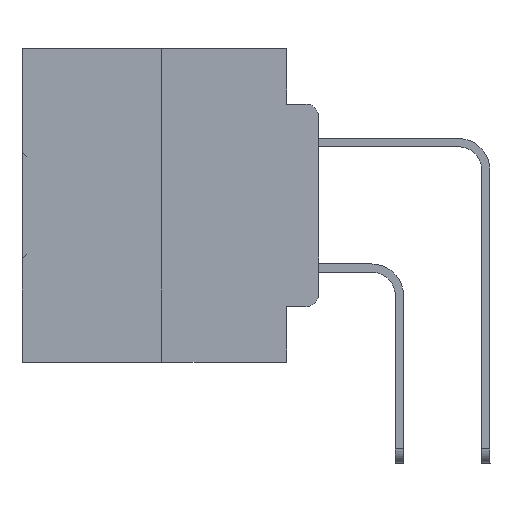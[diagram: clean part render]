
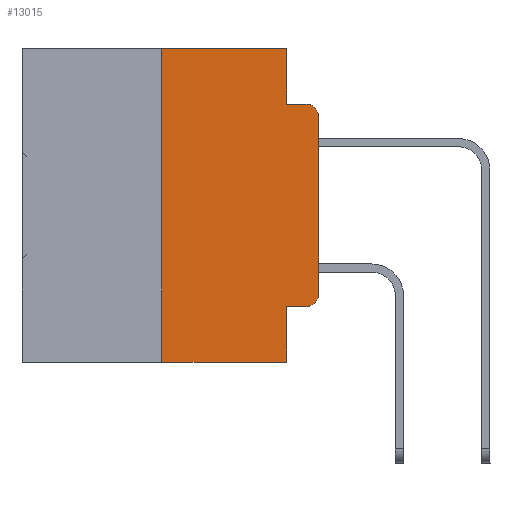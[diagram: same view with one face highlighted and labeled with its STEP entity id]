
A CAD part, left-side view. The second image highlights one B-rep face of the part: STEP entity #13015.
In plain terms, the highlighted planar face has unit normal (-1, 0, 0).
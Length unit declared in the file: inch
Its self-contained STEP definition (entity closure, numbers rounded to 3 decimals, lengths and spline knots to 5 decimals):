
#2 = LINE ( 'NONE', #14968, #14999 ) ;
#311 = DIRECTION ( 'NONE',  ( -1., 0., 0. ) ) ;
#765 = CIRCLE ( 'NONE', #27268, 0.02 ) ;
#953 = FACE_OUTER_BOUND ( 'NONE', #35140, .T. ) ;
#1009 = CARTESIAN_POINT ( 'NONE',  ( 0., 0.051, 0. ) ) ;
#1306 = CARTESIAN_POINT ( 'NONE',  ( 0., 0.051, -0.4115 ) ) ;
#2291 = LINE ( 'NONE', #12641, #8899 ) ;
#2519 = VERTEX_POINT ( 'NONE', #21751 ) ;
#3044 = VERTEX_POINT ( 'NONE', #28728 ) ;
#4275 = ORIENTED_EDGE ( 'NONE', *, *, #31903, .F. ) ;
#4675 = DIRECTION ( 'NONE',  ( 0., -1., 0. ) ) ;
#4697 = AXIS2_PLACEMENT_3D ( 'NONE', #22525, #6016, #25320 ) ;
#4734 = ORIENTED_EDGE ( 'NONE', *, *, #33663, .F. ) ;
#6016 = DIRECTION ( 'NONE',  ( 1., 0., 0. ) ) ;
#6098 = ORIENTED_EDGE ( 'NONE', *, *, #19002, .T. ) ;
#7872 = CARTESIAN_POINT ( 'NONE',  ( 0., 0.051, -0.0885 ) ) ;
#8592 = CARTESIAN_POINT ( 'NONE',  ( 0., 0.051, 0. ) ) ;
#8665 = CARTESIAN_POINT ( 'NONE',  ( 0., 0., -0.3915 ) ) ;
#8899 = VECTOR ( 'NONE', #20821, 39.37008 ) ;
#9166 = VECTOR ( 'NONE', #35363, 39.37008 ) ;
#9259 = EDGE_CURVE ( 'NONE', #13122, #3044, #13547, .T. ) ;
#10264 = CARTESIAN_POINT ( 'NONE',  ( 0., 0.473, -0.5 ) ) ;
#11190 = AXIS2_PLACEMENT_3D ( 'NONE', #17132, #311, #19896 ) ;
#11481 = CARTESIAN_POINT ( 'NONE',  ( 0., 0.02, -0.4115 ) ) ;
#11544 = PLANE ( 'NONE',  #4697 ) ;
#12348 = VECTOR ( 'NONE', #15047, 39.37008 ) ;
#12641 = CARTESIAN_POINT ( 'NONE',  ( 0., 0., 0. ) ) ;
#12862 = CIRCLE ( 'NONE', #11190, 0.02 ) ;
#13015 = ADVANCED_FACE ( 'NONE', ( #953 ), #11544, .F. ) ;
#13122 = VERTEX_POINT ( 'NONE', #1306 ) ;
#13547 = LINE ( 'NONE', #8592, #34394 ) ;
#13906 = CARTESIAN_POINT ( 'NONE',  ( 0., 0.02, -0.1085 ) ) ;
#14566 = EDGE_CURVE ( 'NONE', #28835, #17839, #17956, .T. ) ;
#14968 = CARTESIAN_POINT ( 'NONE',  ( 0., 0.473, 0. ) ) ;
#14999 = VECTOR ( 'NONE', #33939, 39.37008 ) ;
#15027 = VERTEX_POINT ( 'NONE', #11481 ) ;
#15047 = DIRECTION ( 'NONE',  ( 0., 0., -1. ) ) ;
#16044 = VERTEX_POINT ( 'NONE', #32412 ) ;
#16150 = ORIENTED_EDGE ( 'NONE', *, *, #21809, .T. ) ;
#16586 = LINE ( 'NONE', #32496, #9166 ) ;
#16682 = DIRECTION ( 'NONE',  ( 0., 0., -1. ) ) ;
#17132 = CARTESIAN_POINT ( 'NONE',  ( 0., 0.02, -0.3915 ) ) ;
#17839 = VERTEX_POINT ( 'NONE', #7872 ) ;
#17892 = ORIENTED_EDGE ( 'NONE', *, *, #33539, .T. ) ;
#17956 = LINE ( 'NONE', #1009, #12348 ) ;
#18269 = EDGE_CURVE ( 'NONE', #26277, #2519, #2291, .T. ) ;
#19002 = EDGE_CURVE ( 'NONE', #13122, #15027, #29461, .T. ) ;
#19896 = DIRECTION ( 'NONE',  ( 0., 0., -1. ) ) ;
#20504 = VERTEX_POINT ( 'NONE', #31419 ) ;
#20821 = DIRECTION ( 'NONE',  ( 0., 0., 1. ) ) ;
#21751 = CARTESIAN_POINT ( 'NONE',  ( 0., 0., -0.1085 ) ) ;
#21809 = EDGE_CURVE ( 'NONE', #16044, #3044, #35278, .T. ) ;
#21940 = EDGE_CURVE ( 'NONE', #16044, #20504, #16586, .T. ) ;
#22525 = CARTESIAN_POINT ( 'NONE',  ( 0., 0.473, 0. ) ) ;
#22625 = EDGE_CURVE ( 'NONE', #2519, #24199, #765, .T. ) ;
#23136 = VECTOR ( 'NONE', #31879, 39.37008 ) ;
#24061 = CARTESIAN_POINT ( 'NONE',  ( 0., 0.051, -0.0885 ) ) ;
#24199 = VERTEX_POINT ( 'NONE', #29444 ) ;
#24636 = ORIENTED_EDGE ( 'NONE', *, *, #22625, .T. ) ;
#25098 = DIRECTION ( 'NONE',  ( 0., 0., -1. ) ) ;
#25320 = DIRECTION ( 'NONE',  ( 0., 0., -1. ) ) ;
#25516 = ORIENTED_EDGE ( 'NONE', *, *, #9259, .F. ) ;
#26277 = VERTEX_POINT ( 'NONE', #8665 ) ;
#26313 = ORIENTED_EDGE ( 'NONE', *, *, #14566, .F. ) ;
#26567 = CARTESIAN_POINT ( 'NONE',  ( 0., 0.051, -0.4115 ) ) ;
#27268 = AXIS2_PLACEMENT_3D ( 'NONE', #13906, #32917, #16682 ) ;
#28076 = VECTOR ( 'NONE', #29456, 39.37008 ) ;
#28728 = CARTESIAN_POINT ( 'NONE',  ( 0., 0.051, -0.5 ) ) ;
#28835 = VERTEX_POINT ( 'NONE', #31037 ) ;
#29444 = CARTESIAN_POINT ( 'NONE',  ( 0., 0.02, -0.0885 ) ) ;
#29456 = DIRECTION ( 'NONE',  ( 0., -1., 0. ) ) ;
#29461 = LINE ( 'NONE', #26567, #23136 ) ;
#29663 = VECTOR ( 'NONE', #4675, 39.37008 ) ;
#31037 = CARTESIAN_POINT ( 'NONE',  ( 0., 0.051, 0. ) ) ;
#31360 = LINE ( 'NONE', #24061, #29663 ) ;
#31419 = CARTESIAN_POINT ( 'NONE',  ( 0., 0.25, 0. ) ) ;
#31879 = DIRECTION ( 'NONE',  ( 0., -1., 0. ) ) ;
#31903 = EDGE_CURVE ( 'NONE', #17839, #24199, #31360, .T. ) ;
#32412 = CARTESIAN_POINT ( 'NONE',  ( 0., 0.25, -0.5 ) ) ;
#32496 = CARTESIAN_POINT ( 'NONE',  ( 0., 0.25, 0. ) ) ;
#32612 = ORIENTED_EDGE ( 'NONE', *, *, #18269, .T. ) ;
#32673 = ORIENTED_EDGE ( 'NONE', *, *, #21940, .F. ) ;
#32917 = DIRECTION ( 'NONE',  ( -1., 0., 0. ) ) ;
#33539 = EDGE_CURVE ( 'NONE', #15027, #26277, #12862, .T. ) ;
#33663 = EDGE_CURVE ( 'NONE', #20504, #28835, #2, .T. ) ;
#33939 = DIRECTION ( 'NONE',  ( 0., -1., 0. ) ) ;
#34394 = VECTOR ( 'NONE', #25098, 39.37008 ) ;
#35140 = EDGE_LOOP ( 'NONE', ( #32612, #24636, #4275, #26313, #4734, #32673, #16150, #25516, #6098, #17892 ) ) ;
#35278 = LINE ( 'NONE', #10264, #28076 ) ;
#35363 = DIRECTION ( 'NONE',  ( 0., 0., 1. ) ) ;
